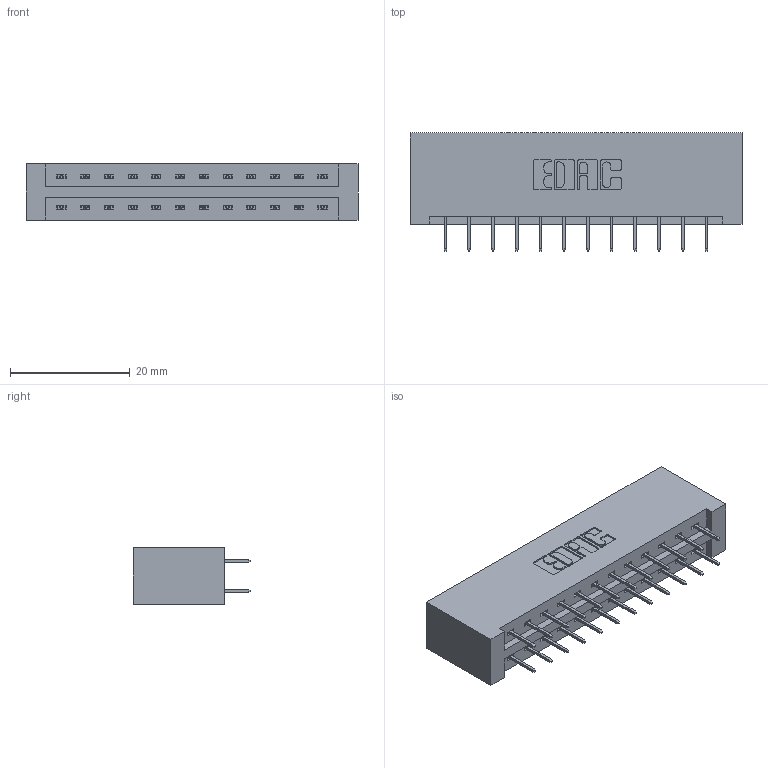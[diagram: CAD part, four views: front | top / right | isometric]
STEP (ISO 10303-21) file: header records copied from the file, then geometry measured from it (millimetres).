
FILE_DESCRIPTION (( 'STEP AP203' ), '1' );
FILE_NAME ('387-024-524-201.STEP', '2019-10-16T18:02:12', ( '' ), ( '' ), 'SwSTEP 2.0', 'SolidWorks 2016', '' );
FILE_SCHEMA (( 'CONFIG_CONTROL_DESIGN' ));
Length unit declared in the file: inch
Products named in the file (3): 345-292-001_345-293-124; 387-024-524-201; 337 Part_No Mounting Lugs
Assembly tree (25 placements, depth 2):
  387-024-524-201
    337 Part_No Mounting Lugs
    345-292-001_345-293-124  x24
Bounding box: 55.42 x 19.69 x 9.4 mm (x, y, z)
Volume: 6166 mm3; surface area: 6622.9 mm2
Topology: 25 solids, 25 shells, 1498 faces, 4247 edges, 2734 vertices
Faces by surface type: plane 1122, cylinder 376
Entity records: 12981 total; most frequent: CARTESIAN_POINT 2210, ORIENTED_EDGE 2146, DIRECTION 1929, EDGE_CURVE 1073, VECTOR 957, LINE 957, VERTEX_POINT 710, AXIS2_PLACEMENT_3D 486
